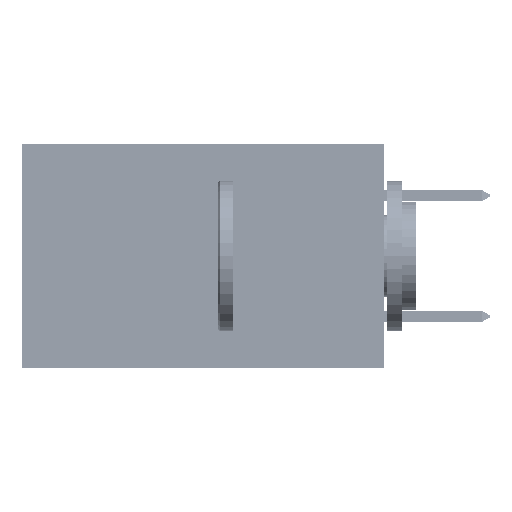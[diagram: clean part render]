
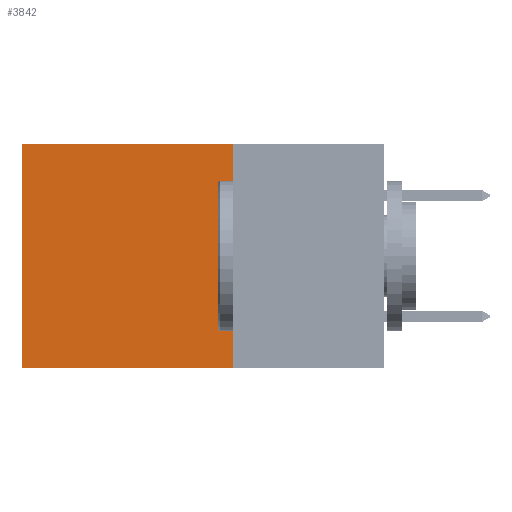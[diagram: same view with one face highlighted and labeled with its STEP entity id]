
A CAD part, left-side view. The second image highlights one B-rep face of the part: STEP entity #3842.
In plain terms, the highlighted planar face has unit normal (-1, 0, 0).
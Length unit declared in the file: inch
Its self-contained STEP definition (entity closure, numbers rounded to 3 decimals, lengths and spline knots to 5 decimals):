
#8 = CARTESIAN_POINT ( 'NONE',  ( 0.2875, 0.6, 0. ) ) ;
#3842 = ADVANCED_FACE ( 'NONE', ( #5788 ), #34217, .F. ) ;
#5788 = FACE_OUTER_BOUND ( 'NONE', #37739, .T. ) ;
#6148 = ORIENTED_EDGE ( 'NONE', *, *, #7813, .T. ) ;
#6678 = VERTEX_POINT ( 'NONE', #18536 ) ;
#7069 = CARTESIAN_POINT ( 'NONE',  ( 0.2875, 0.25, -0.37 ) ) ;
#7813 = EDGE_CURVE ( 'NONE', #6678, #16689, #9910, .T. ) ;
#9853 = CARTESIAN_POINT ( 'NONE',  ( 0.2875, 0.25, -0.37 ) ) ;
#9910 = LINE ( 'NONE', #14582, #44226 ) ;
#12265 = AXIS2_PLACEMENT_3D ( 'NONE', #30637, #44738, #13104 ) ;
#13104 = DIRECTION ( 'NONE',  ( 0., 0., -1. ) ) ;
#14582 = CARTESIAN_POINT ( 'NONE',  ( 0.2875, 0.25, 0. ) ) ;
#14594 = DIRECTION ( 'NONE',  ( 0., 0., -1. ) ) ;
#16689 = VERTEX_POINT ( 'NONE', #17757 ) ;
#17757 = CARTESIAN_POINT ( 'NONE',  ( 0.2875, 0.6, 0. ) ) ;
#18536 = CARTESIAN_POINT ( 'NONE',  ( 0.2875, 0.25, 0. ) ) ;
#22001 = VERTEX_POINT ( 'NONE', #9853 ) ;
#22119 = VECTOR ( 'NONE', #45971, 39.37008 ) ;
#25818 = EDGE_CURVE ( 'NONE', #16689, #36088, #40715, .T. ) ;
#28715 = ORIENTED_EDGE ( 'NONE', *, *, #41607, .F. ) ;
#30637 = CARTESIAN_POINT ( 'NONE',  ( 0.2875, 0.25, 0. ) ) ;
#30685 = EDGE_CURVE ( 'NONE', #6678, #22001, #35251, .T. ) ;
#31301 = VECTOR ( 'NONE', #14594, 39.37008 ) ;
#34217 = PLANE ( 'NONE',  #12265 ) ;
#34223 = CARTESIAN_POINT ( 'NONE',  ( 0.2875, 0.25, 0. ) ) ;
#35251 = LINE ( 'NONE', #34223, #43527 ) ;
#36088 = VERTEX_POINT ( 'NONE', #45549 ) ;
#37739 = EDGE_LOOP ( 'NONE', ( #41987, #28715, #40255, #6148 ) ) ;
#40255 = ORIENTED_EDGE ( 'NONE', *, *, #30685, .F. ) ;
#40715 = LINE ( 'NONE', #8, #31301 ) ;
#41164 = DIRECTION ( 'NONE',  ( 0., 0., -1. ) ) ;
#41607 = EDGE_CURVE ( 'NONE', #22001, #36088, #41983, .T. ) ;
#41983 = LINE ( 'NONE', #7069, #22119 ) ;
#41987 = ORIENTED_EDGE ( 'NONE', *, *, #25818, .T. ) ;
#42808 = DIRECTION ( 'NONE',  ( 0., 1., 0. ) ) ;
#43527 = VECTOR ( 'NONE', #41164, 39.37008 ) ;
#44226 = VECTOR ( 'NONE', #42808, 39.37008 ) ;
#44738 = DIRECTION ( 'NONE',  ( 1., 0., 0. ) ) ;
#45549 = CARTESIAN_POINT ( 'NONE',  ( 0.2875, 0.6, -0.37 ) ) ;
#45971 = DIRECTION ( 'NONE',  ( 0., 1., 0. ) ) ;
